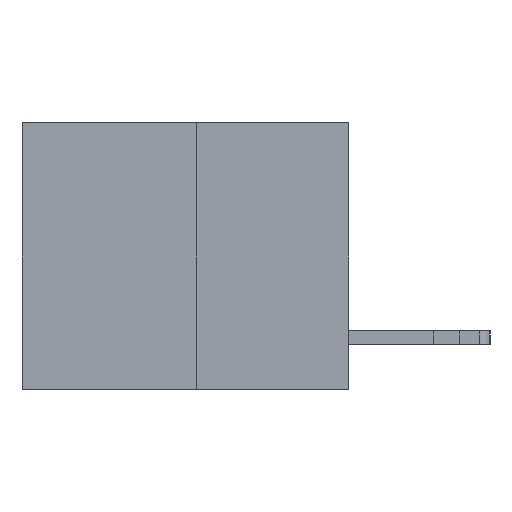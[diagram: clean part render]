
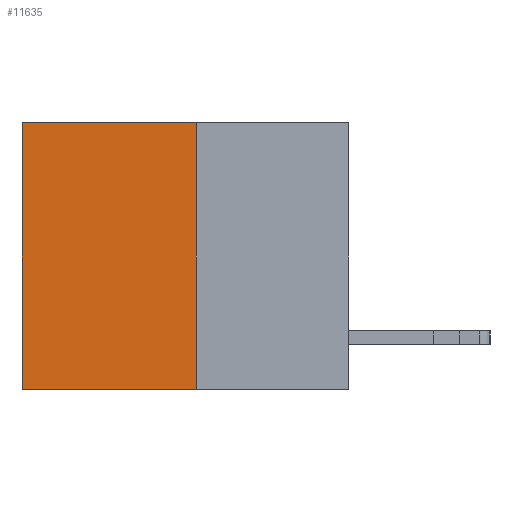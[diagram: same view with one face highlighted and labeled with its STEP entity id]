
A CAD part, left-side view. The second image highlights one B-rep face of the part: STEP entity #11635.
In plain terms, the highlighted planar face has unit normal (-1, 0, 0).
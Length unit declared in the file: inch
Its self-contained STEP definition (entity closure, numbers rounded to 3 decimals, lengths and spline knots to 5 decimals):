
#131 = VECTOR ( 'NONE', #4370, 39.37008 ) ;
#827 = VERTEX_POINT ( 'NONE', #3179 ) ;
#1965 = VERTEX_POINT ( 'NONE', #8312 ) ;
#2116 = DIRECTION ( 'NONE',  ( 0., 1., 0. ) ) ;
#2541 = EDGE_CURVE ( 'NONE', #12288, #827, #4681, .T. ) ;
#2768 = LINE ( 'NONE', #15200, #131 ) ;
#2958 = DIRECTION ( 'NONE',  ( 0., 0., -1. ) ) ;
#3179 = CARTESIAN_POINT ( 'NONE',  ( 0.3165, 0.6, 0. ) ) ;
#3263 = CARTESIAN_POINT ( 'NONE',  ( 0.3165, 0.6, -0.49 ) ) ;
#3576 = VECTOR ( 'NONE', #5806, 39.37008 ) ;
#4370 = DIRECTION ( 'NONE',  ( 0., 1., 0. ) ) ;
#4460 = CARTESIAN_POINT ( 'NONE',  ( 0.3165, 0.28, 0. ) ) ;
#4562 = EDGE_CURVE ( 'NONE', #11299, #1965, #2768, .T. ) ;
#4681 = LINE ( 'NONE', #4460, #13061 ) ;
#4797 = AXIS2_PLACEMENT_3D ( 'NONE', #7303, #4922, #13266 ) ;
#4922 = DIRECTION ( 'NONE',  ( 1., 0., 0. ) ) ;
#5297 = CARTESIAN_POINT ( 'NONE',  ( 0.3165, 0.28, -0.49 ) ) ;
#5806 = DIRECTION ( 'NONE',  ( 0., 0., -1. ) ) ;
#5915 = ORIENTED_EDGE ( 'NONE', *, *, #4562, .F. ) ;
#5937 = EDGE_LOOP ( 'NONE', ( #8709, #5915, #8552, #13517 ) ) ;
#6265 = CARTESIAN_POINT ( 'NONE',  ( 0.3165, 0.28, 0. ) ) ;
#6534 = EDGE_CURVE ( 'NONE', #827, #1965, #13497, .T. ) ;
#7303 = CARTESIAN_POINT ( 'NONE',  ( 0.3165, 0.28, -0.49 ) ) ;
#8287 = EDGE_CURVE ( 'NONE', #12288, #11299, #8323, .T. ) ;
#8312 = CARTESIAN_POINT ( 'NONE',  ( 0.3165, 0.6, -0.49 ) ) ;
#8323 = LINE ( 'NONE', #10173, #9241 ) ;
#8552 = ORIENTED_EDGE ( 'NONE', *, *, #8287, .F. ) ;
#8709 = ORIENTED_EDGE ( 'NONE', *, *, #6534, .T. ) ;
#9241 = VECTOR ( 'NONE', #2958, 39.37008 ) ;
#9635 = PLANE ( 'NONE',  #4797 ) ;
#10173 = CARTESIAN_POINT ( 'NONE',  ( 0.3165, 0.28, -0.49 ) ) ;
#11299 = VERTEX_POINT ( 'NONE', #5297 ) ;
#11635 = ADVANCED_FACE ( 'NONE', ( #15199 ), #9635, .F. ) ;
#12288 = VERTEX_POINT ( 'NONE', #6265 ) ;
#13061 = VECTOR ( 'NONE', #2116, 39.37008 ) ;
#13266 = DIRECTION ( 'NONE',  ( 0., 0., -1. ) ) ;
#13497 = LINE ( 'NONE', #3263, #3576 ) ;
#13517 = ORIENTED_EDGE ( 'NONE', *, *, #2541, .T. ) ;
#15199 = FACE_OUTER_BOUND ( 'NONE', #5937, .T. ) ;
#15200 = CARTESIAN_POINT ( 'NONE',  ( 0.3165, 0.28, -0.49 ) ) ;
